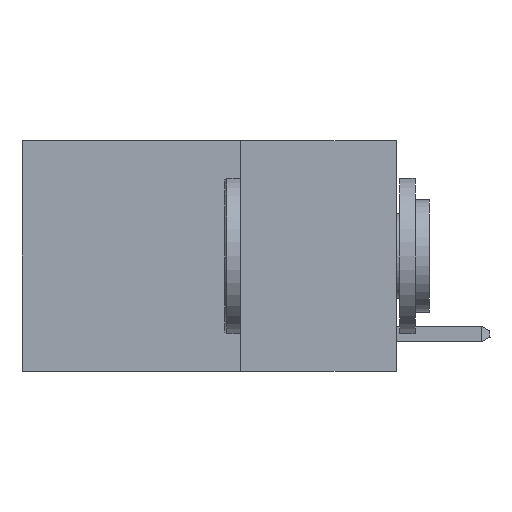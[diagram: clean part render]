
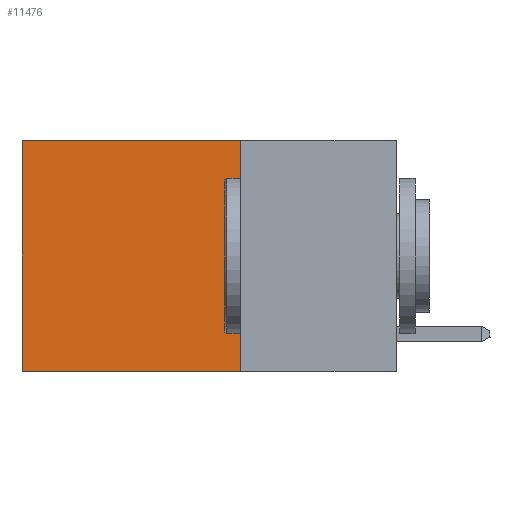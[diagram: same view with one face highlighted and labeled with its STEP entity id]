
A CAD part, left-side view. The second image highlights one B-rep face of the part: STEP entity #11476.
In plain terms, the highlighted planar face has unit normal (-1, 0, 0).
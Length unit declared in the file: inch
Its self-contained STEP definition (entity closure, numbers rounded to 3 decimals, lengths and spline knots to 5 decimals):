
#671 = DIRECTION ( 'NONE',  ( 0., 0., -1. ) ) ;
#1747 = DIRECTION ( 'NONE',  ( 1., 0., 0. ) ) ;
#2180 = ORIENTED_EDGE ( 'NONE', *, *, #26811, .F. ) ;
#2934 = EDGE_CURVE ( 'NONE', #20005, #23662, #21690, .T. ) ;
#3608 = AXIS2_PLACEMENT_3D ( 'NONE', #11169, #1747, #18248 ) ;
#5070 = ORIENTED_EDGE ( 'NONE', *, *, #28608, .F. ) ;
#6658 = LINE ( 'NONE', #25639, #18381 ) ;
#7232 = DIRECTION ( 'NONE',  ( 0., 0., -1. ) ) ;
#8148 = VECTOR ( 'NONE', #8406, 39.37008 ) ;
#8406 = DIRECTION ( 'NONE',  ( 0., 1., 0. ) ) ;
#10105 = ORIENTED_EDGE ( 'NONE', *, *, #2934, .T. ) ;
#11169 = CARTESIAN_POINT ( 'NONE',  ( 0.2625, 0.25, 0. ) ) ;
#11476 = ADVANCED_FACE ( 'NONE', ( #22411 ), #15915, .F. ) ;
#11814 = DIRECTION ( 'NONE',  ( 0., 1., 0. ) ) ;
#12396 = VERTEX_POINT ( 'NONE', #16954 ) ;
#13048 = ORIENTED_EDGE ( 'NONE', *, *, #16074, .T. ) ;
#13657 = VERTEX_POINT ( 'NONE', #21615 ) ;
#15760 = CARTESIAN_POINT ( 'NONE',  ( 0.2625, 0.6, 0. ) ) ;
#15915 = PLANE ( 'NONE',  #3608 ) ;
#16074 = EDGE_CURVE ( 'NONE', #13657, #20005, #6658, .T. ) ;
#16549 = CARTESIAN_POINT ( 'NONE',  ( 0.2625, 0.25, 0. ) ) ;
#16954 = CARTESIAN_POINT ( 'NONE',  ( 0.2625, 0.25, -0.37 ) ) ;
#18248 = DIRECTION ( 'NONE',  ( 0., 0., -1. ) ) ;
#18381 = VECTOR ( 'NONE', #11814, 39.37008 ) ;
#19486 = CARTESIAN_POINT ( 'NONE',  ( 0.2625, 0.6, -0.37 ) ) ;
#19864 = LINE ( 'NONE', #20053, #8148 ) ;
#20005 = VERTEX_POINT ( 'NONE', #15760 ) ;
#20053 = CARTESIAN_POINT ( 'NONE',  ( 0.2625, 0.25, -0.37 ) ) ;
#20970 = VECTOR ( 'NONE', #671, 39.37008 ) ;
#21615 = CARTESIAN_POINT ( 'NONE',  ( 0.2625, 0.25, 0. ) ) ;
#21690 = LINE ( 'NONE', #28576, #20970 ) ;
#22411 = FACE_OUTER_BOUND ( 'NONE', #28516, .T. ) ;
#22576 = VECTOR ( 'NONE', #7232, 39.37008 ) ;
#23662 = VERTEX_POINT ( 'NONE', #19486 ) ;
#25639 = CARTESIAN_POINT ( 'NONE',  ( 0.2625, 0.25, 0. ) ) ;
#26811 = EDGE_CURVE ( 'NONE', #12396, #23662, #19864, .T. ) ;
#28516 = EDGE_LOOP ( 'NONE', ( #10105, #2180, #5070, #13048 ) ) ;
#28576 = CARTESIAN_POINT ( 'NONE',  ( 0.2625, 0.6, 0. ) ) ;
#28608 = EDGE_CURVE ( 'NONE', #13657, #12396, #28624, .T. ) ;
#28624 = LINE ( 'NONE', #16549, #22576 ) ;
